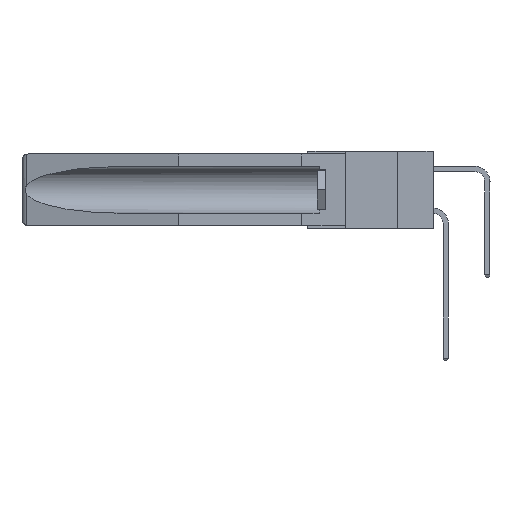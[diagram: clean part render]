
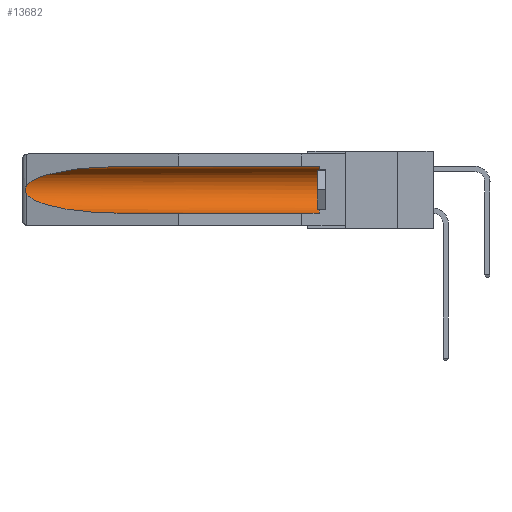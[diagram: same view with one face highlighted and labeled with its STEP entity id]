
A CAD part, left-side view. The second image highlights one B-rep face of the part: STEP entity #13682.
In plain terms, the highlighted cylindrical face has radius 2.857 mm (diameter 5.715 mm), a partial arc.
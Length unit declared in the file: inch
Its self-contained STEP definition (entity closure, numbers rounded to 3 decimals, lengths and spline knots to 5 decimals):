
#359 =( BOUNDED_CURVE ( )  B_SPLINE_CURVE ( 3, ( #15899, #24497, #11953, #7258 ),
 .UNSPECIFIED., .F., .F. ) 
 B_SPLINE_CURVE_WITH_KNOTS ( ( 4, 4 ),
 ( 4.71239, 6.08839 ),
 .UNSPECIFIED. ) 
 CURVE ( )  GEOMETRIC_REPRESENTATION_ITEM ( )  RATIONAL_B_SPLINE_CURVE ( ( 1., 0.848, 0.848, 1. ) ) 
 REPRESENTATION_ITEM ( '' )  );
#360 = CARTESIAN_POINT ( 'NONE',  ( 0.155, 0.126, -0.1715 ) ) ;
#1553 = CARTESIAN_POINT ( 'NONE',  ( 0.155, 0.126, -0.284 ) ) ;
#1753 = CARTESIAN_POINT ( 'NONE',  ( 0.155, 0.126, -0.059 ) ) ;
#1981 = ORIENTED_EDGE ( 'NONE', *, *, #8961, .F. ) ;
#2396 = AXIS2_PLACEMENT_3D ( 'NONE', #15289, #15477, #15570 ) ;
#2940 = LINE ( 'NONE', #6221, #21785 ) ;
#3955 = CARTESIAN_POINT ( 'NONE',  ( 0.26597, 1.52961, -0.15275 ) ) ;
#6221 = CARTESIAN_POINT ( 'NONE',  ( 0.155, -0.30754, -0.284 ) ) ;
#6273 = VERTEX_POINT ( 'NONE', #12949 ) ;
#6379 = B_SPLINE_CURVE_WITH_KNOTS ( 'NONE', 3,
 ( #14942, #3955, #17032, #8290, #25493, #10725, #27664, #14760, #12716, #12812 ),
 .UNSPECIFIED., .F., .F.,
 ( 4, 2, 2, 2, 4 ),
 ( 0., 0.00029, 0.00058, 0.00087, 0.00117 ),
 .UNSPECIFIED. ) ;
#6762 = DIRECTION ( 'NONE',  ( 0., -1., 0. ) ) ;
#6814 = VERTEX_POINT ( 'NONE', #9297 ) ;
#7258 = CARTESIAN_POINT ( 'NONE',  ( 0.26537, 1.52718, -0.14972 ) ) ;
#7997 = CARTESIAN_POINT ( 'NONE',  ( 0.26537, 1.52718, -0.19328 ) ) ;
#8280 = ORIENTED_EDGE ( 'NONE', *, *, #22853, .T. ) ;
#8290 = CARTESIAN_POINT ( 'NONE',  ( 0.2673, 1.5327, -0.16383 ) ) ;
#8961 = EDGE_CURVE ( 'NONE', #20372, #6814, #2940, .T. ) ;
#9297 = CARTESIAN_POINT ( 'NONE',  ( 0.155, 1.07973, -0.284 ) ) ;
#10725 = CARTESIAN_POINT ( 'NONE',  ( 0.2675, 1.53308, -0.17534 ) ) ;
#11694 = EDGE_CURVE ( 'NONE', #24190, #15977, #359, .T. ) ;
#11845 = EDGE_CURVE ( 'NONE', #6273, #6814, #17978, .T. ) ;
#11879 = CARTESIAN_POINT ( 'NONE',  ( 0.155, -0.30754, -0.059 ) ) ;
#11953 = CARTESIAN_POINT ( 'NONE',  ( 0.25451, 1.48313, -0.09465 ) ) ;
#12716 = CARTESIAN_POINT ( 'NONE',  ( 0.26597, 1.5296, -0.19026 ) ) ;
#12812 = CARTESIAN_POINT ( 'NONE',  ( 0.26537, 1.52718, -0.19328 ) ) ;
#12926 = EDGE_CURVE ( 'NONE', #25915, #24190, #18426, .T. ) ;
#12949 = CARTESIAN_POINT ( 'NONE',  ( 0.26537, 1.52718, -0.19328 ) ) ;
#13682 = ADVANCED_FACE ( 'NONE', ( #21050 ), #27483, .F. ) ;
#14551 = CARTESIAN_POINT ( 'NONE',  ( 0.26537, 1.52718, -0.14972 ) ) ;
#14760 = CARTESIAN_POINT ( 'NONE',  ( 0.26655, 1.53094, -0.18657 ) ) ;
#14942 = CARTESIAN_POINT ( 'NONE',  ( 0.26537, 1.52718, -0.14972 ) ) ;
#15289 = CARTESIAN_POINT ( 'NONE',  ( 0.155, -0.30754, -0.1715 ) ) ;
#15418 = DIRECTION ( 'NONE',  ( 0., 0., 1. ) ) ;
#15477 = DIRECTION ( 'NONE',  ( 0., 1., 0. ) ) ;
#15570 = DIRECTION ( 'NONE',  ( 0., 0., 1. ) ) ;
#15854 = AXIS2_PLACEMENT_3D ( 'NONE', #360, #6762, #15418 ) ;
#15899 = CARTESIAN_POINT ( 'NONE',  ( 0.155, 1.07973, -0.059 ) ) ;
#15909 = CARTESIAN_POINT ( 'NONE',  ( 0.155, 1.07973, -0.059 ) ) ;
#15977 = VERTEX_POINT ( 'NONE', #14551 ) ;
#16861 = DIRECTION ( 'NONE',  ( 0., 1., 0. ) ) ;
#17032 = CARTESIAN_POINT ( 'NONE',  ( 0.26654, 1.53092, -0.15636 ) ) ;
#17638 = EDGE_LOOP ( 'NONE', ( #27301, #8280, #21996, #1981, #27714, #25729 ) ) ;
#17978 =( BOUNDED_CURVE ( )  B_SPLINE_CURVE ( 3, ( #7997, #25206, #18818, #25027 ),
 .UNSPECIFIED., .F., .F. ) 
 B_SPLINE_CURVE_WITH_KNOTS ( ( 4, 4 ),
 ( 0.1948, 1.5708 ),
 .UNSPECIFIED. ) 
 CURVE ( )  GEOMETRIC_REPRESENTATION_ITEM ( )  RATIONAL_B_SPLINE_CURVE ( ( 1., 0.848, 0.848, 1. ) ) 
 REPRESENTATION_ITEM ( '' )  );
#18426 = LINE ( 'NONE', #11879, #19775 ) ;
#18818 = CARTESIAN_POINT ( 'NONE',  ( 0.21114, 1.30732, -0.284 ) ) ;
#19775 = VECTOR ( 'NONE', #27138, 39.37008 ) ;
#19944 = CIRCLE ( 'NONE', #15854, 0.1125 ) ;
#20372 = VERTEX_POINT ( 'NONE', #1553 ) ;
#21050 = FACE_OUTER_BOUND ( 'NONE', #17638, .T. ) ;
#21785 = VECTOR ( 'NONE', #16861, 39.37008 ) ;
#21996 = ORIENTED_EDGE ( 'NONE', *, *, #11845, .T. ) ;
#22853 = EDGE_CURVE ( 'NONE', #15977, #6273, #6379, .T. ) ;
#24190 = VERTEX_POINT ( 'NONE', #15909 ) ;
#24497 = CARTESIAN_POINT ( 'NONE',  ( 0.21114, 1.30732, -0.059 ) ) ;
#25027 = CARTESIAN_POINT ( 'NONE',  ( 0.155, 1.07973, -0.284 ) ) ;
#25206 = CARTESIAN_POINT ( 'NONE',  ( 0.25451, 1.48313, -0.24835 ) ) ;
#25493 = CARTESIAN_POINT ( 'NONE',  ( 0.2675, 1.53308, -0.16763 ) ) ;
#25729 = ORIENTED_EDGE ( 'NONE', *, *, #12926, .T. ) ;
#25915 = VERTEX_POINT ( 'NONE', #1753 ) ;
#26162 = EDGE_CURVE ( 'NONE', #20372, #25915, #19944, .T. ) ;
#27138 = DIRECTION ( 'NONE',  ( 0., 1., 0. ) ) ;
#27301 = ORIENTED_EDGE ( 'NONE', *, *, #11694, .T. ) ;
#27483 = CYLINDRICAL_SURFACE ( 'NONE', #2396, 0.1125 ) ;
#27664 = CARTESIAN_POINT ( 'NONE',  ( 0.2673, 1.53269, -0.17917 ) ) ;
#27714 = ORIENTED_EDGE ( 'NONE', *, *, #26162, .T. ) ;
